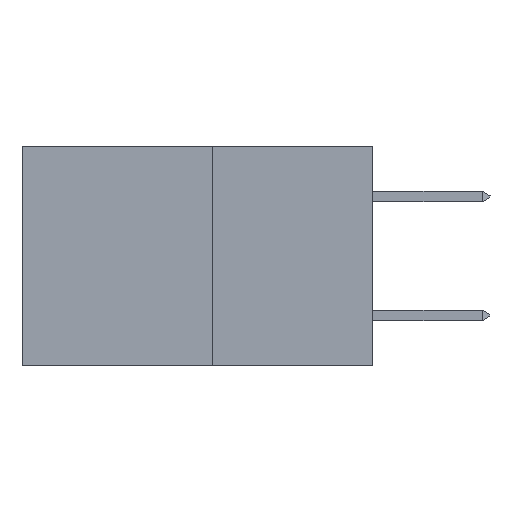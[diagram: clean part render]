
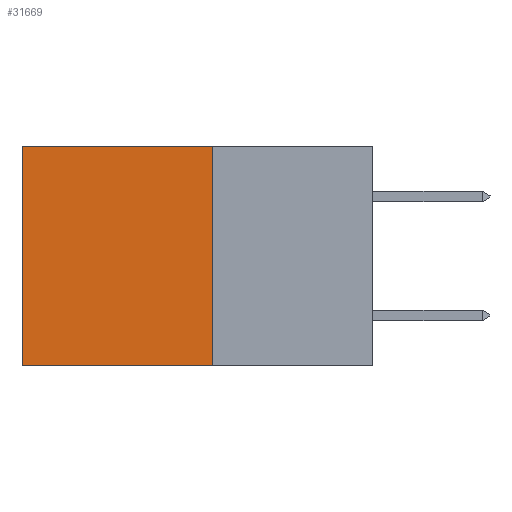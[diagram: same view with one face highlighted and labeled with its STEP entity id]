
A CAD part, left-side view. The second image highlights one B-rep face of the part: STEP entity #31669.
In plain terms, the highlighted planar face has unit normal (-1, 0, 0).
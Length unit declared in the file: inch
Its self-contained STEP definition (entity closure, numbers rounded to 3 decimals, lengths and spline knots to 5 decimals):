
#461 = LINE ( 'NONE', #20935, #27903 ) ;
#1690 = ORIENTED_EDGE ( 'NONE', *, *, #33465, .T. ) ;
#2279 = DIRECTION ( 'NONE',  ( 1., 0., 0. ) ) ;
#7111 = EDGE_CURVE ( 'NONE', #10733, #19712, #461, .T. ) ;
#9645 = DIRECTION ( 'NONE',  ( 0., 0., -1. ) ) ;
#10018 = EDGE_CURVE ( 'NONE', #28391, #10733, #15772, .T. ) ;
#10733 = VERTEX_POINT ( 'NONE', #28130 ) ;
#11376 = VERTEX_POINT ( 'NONE', #14688 ) ;
#14196 = VECTOR ( 'NONE', #9645, 39.37008 ) ;
#14270 = ORIENTED_EDGE ( 'NONE', *, *, #30332, .T. ) ;
#14688 = CARTESIAN_POINT ( 'NONE',  ( 0.277, 0.59, 0. ) ) ;
#14834 = DIRECTION ( 'NONE',  ( 0., 0., -1. ) ) ;
#15772 = LINE ( 'NONE', #33143, #28104 ) ;
#15846 = CARTESIAN_POINT ( 'NONE',  ( 0.277, 0.27, 0. ) ) ;
#17708 = AXIS2_PLACEMENT_3D ( 'NONE', #18338, #2279, #20972 ) ;
#18338 = CARTESIAN_POINT ( 'NONE',  ( 0.277, 0.27, -0.37 ) ) ;
#18523 = DIRECTION ( 'NONE',  ( 0., 1., 0. ) ) ;
#19079 = DIRECTION ( 'NONE',  ( 0., 1., 0. ) ) ;
#19712 = VERTEX_POINT ( 'NONE', #29522 ) ;
#20827 = EDGE_LOOP ( 'NONE', ( #1690, #28106, #27036, #14270 ) ) ;
#20935 = CARTESIAN_POINT ( 'NONE',  ( 0.277, 0.27, -0.37 ) ) ;
#20952 = LINE ( 'NONE', #15846, #34102 ) ;
#20972 = DIRECTION ( 'NONE',  ( 0., 0., -1. ) ) ;
#22970 = CARTESIAN_POINT ( 'NONE',  ( 0.277, 0.59, -0.37 ) ) ;
#27036 = ORIENTED_EDGE ( 'NONE', *, *, #10018, .F. ) ;
#27903 = VECTOR ( 'NONE', #19079, 39.37008 ) ;
#27938 = CARTESIAN_POINT ( 'NONE',  ( 0.277, 0.27, 0. ) ) ;
#28104 = VECTOR ( 'NONE', #14834, 39.37008 ) ;
#28106 = ORIENTED_EDGE ( 'NONE', *, *, #7111, .F. ) ;
#28130 = CARTESIAN_POINT ( 'NONE',  ( 0.277, 0.27, -0.37 ) ) ;
#28195 = LINE ( 'NONE', #22970, #14196 ) ;
#28391 = VERTEX_POINT ( 'NONE', #27938 ) ;
#28745 = PLANE ( 'NONE',  #17708 ) ;
#29522 = CARTESIAN_POINT ( 'NONE',  ( 0.277, 0.59, -0.37 ) ) ;
#30332 = EDGE_CURVE ( 'NONE', #28391, #11376, #20952, .T. ) ;
#31669 = ADVANCED_FACE ( 'NONE', ( #33700 ), #28745, .F. ) ;
#33143 = CARTESIAN_POINT ( 'NONE',  ( 0.277, 0.27, -0.37 ) ) ;
#33465 = EDGE_CURVE ( 'NONE', #11376, #19712, #28195, .T. ) ;
#33700 = FACE_OUTER_BOUND ( 'NONE', #20827, .T. ) ;
#34102 = VECTOR ( 'NONE', #18523, 39.37008 ) ;
